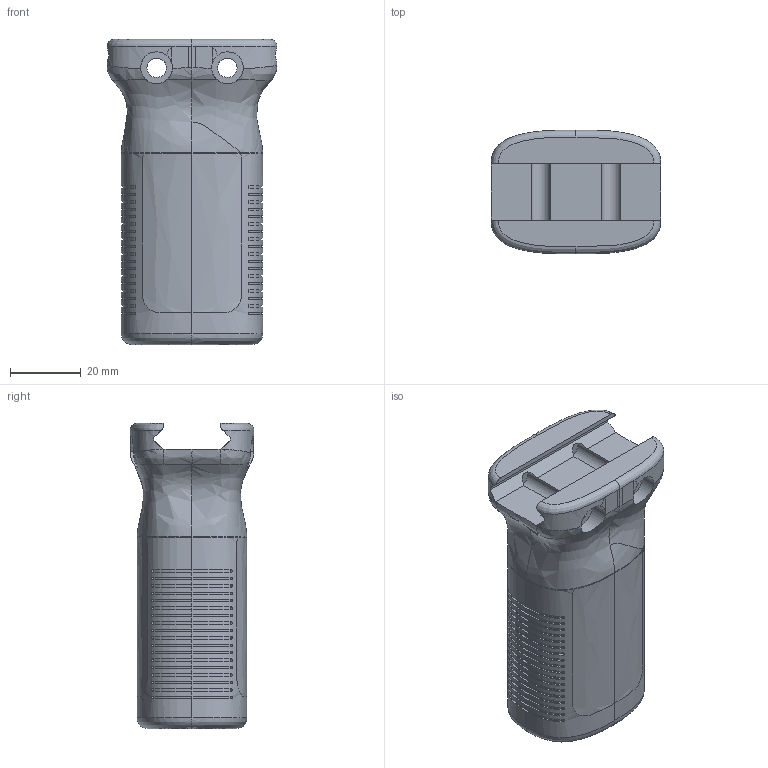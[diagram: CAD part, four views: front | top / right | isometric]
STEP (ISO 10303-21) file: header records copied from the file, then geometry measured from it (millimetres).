
FILE_DESCRIPTION (( 'STEP AP214' ), '1' );
FILE_NAME ('FOSSCAD_RVG_Vertical_Grip.STEP', '2015-04-02T18:58:38', ( 'WarFairy' ), ( '' ), 'SwSTEP 2.0', 'SolidWorks 2013', '' );
FILE_SCHEMA (( 'AUTOMOTIVE_DESIGN' ));
Length unit declared in the file: millimetre
Products named in the file (1): FOSSCAD_RVG_Vertical_Grip
Bounding box: 48 x 35 x 86.25 mm (x, y, z)
Volume: 49324.8 mm3; surface area: 20907.9 mm2
Topology: 1 solids, 1 shells, 434 faces, 1302 edges, 865 vertices
Faces by surface type: bspline 175, cylinder 152, plane 107
Entity records: 27552 total; most frequent: CARTESIAN_POINT 18095, ORIENTED_EDGE 2596, EDGE_CURVE 1298, DIRECTION 965, B_SPLINE_CURVE_WITH_KNOTS 875, VERTEX_POINT 865, EDGE_LOOP 441, ADVANCED_FACE 434
